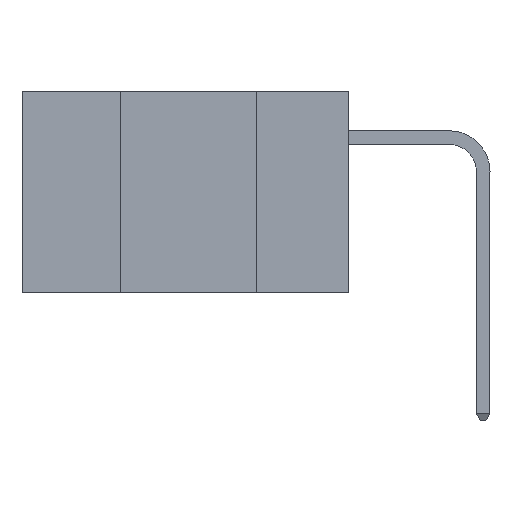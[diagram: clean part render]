
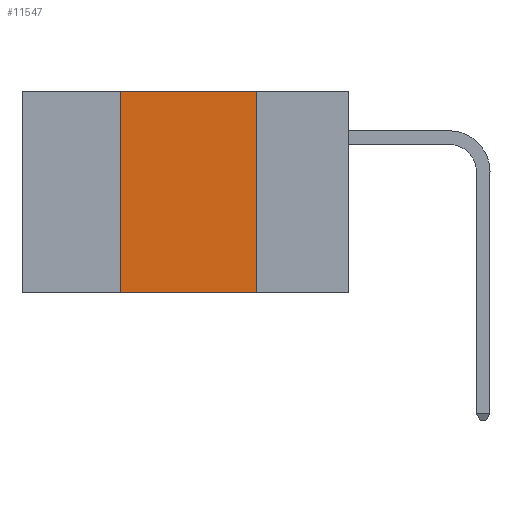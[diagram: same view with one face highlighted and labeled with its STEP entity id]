
A CAD part, left-side view. The second image highlights one B-rep face of the part: STEP entity #11547.
In plain terms, the highlighted planar face has unit normal (-1, 0, 0).
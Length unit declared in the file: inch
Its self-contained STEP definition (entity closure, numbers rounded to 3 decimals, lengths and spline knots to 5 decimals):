
#123 = CARTESIAN_POINT ( 'NONE',  ( 0., 0.42, -0.37 ) ) ;
#1362 = EDGE_LOOP ( 'NONE', ( #5322, #5265, #21734, #24463 ) ) ;
#3909 = EDGE_CURVE ( 'NONE', #28361, #12414, #17825, .T. ) ;
#4504 = CARTESIAN_POINT ( 'NONE',  ( 0., 0.17, 0. ) ) ;
#5265 = ORIENTED_EDGE ( 'NONE', *, *, #24788, .F. ) ;
#5299 = DIRECTION ( 'NONE',  ( 0., -1., 0. ) ) ;
#5322 = ORIENTED_EDGE ( 'NONE', *, *, #19753, .F. ) ;
#5754 = LINE ( 'NONE', #4504, #25176 ) ;
#6226 = DIRECTION ( 'NONE',  ( 0., 0., -1. ) ) ;
#8968 = VECTOR ( 'NONE', #5299, 39.37008 ) ;
#9313 = LINE ( 'NONE', #18518, #18513 ) ;
#11547 = ADVANCED_FACE ( 'NONE', ( #25370 ), #17026, .F. ) ;
#11687 = VERTEX_POINT ( 'NONE', #18327 ) ;
#12092 = DIRECTION ( 'NONE',  ( 0., -1., 0. ) ) ;
#12147 = CARTESIAN_POINT ( 'NONE',  ( 0., 0.42, 0. ) ) ;
#12414 = VERTEX_POINT ( 'NONE', #16113 ) ;
#12415 = CARTESIAN_POINT ( 'NONE',  ( 0., 0.17, 0. ) ) ;
#12488 = EDGE_CURVE ( 'NONE', #28361, #11687, #12990, .T. ) ;
#12990 = LINE ( 'NONE', #12147, #13978 ) ;
#13978 = VECTOR ( 'NONE', #16512, 39.37008 ) ;
#16113 = CARTESIAN_POINT ( 'NONE',  ( 0., 0.17, -0.37 ) ) ;
#16512 = DIRECTION ( 'NONE',  ( 0., 0., 1. ) ) ;
#17026 = PLANE ( 'NONE',  #27450 ) ;
#17231 = DIRECTION ( 'NONE',  ( 1., 0., 0. ) ) ;
#17825 = LINE ( 'NONE', #28169, #8968 ) ;
#18327 = CARTESIAN_POINT ( 'NONE',  ( 0., 0.42, 0. ) ) ;
#18513 = VECTOR ( 'NONE', #12092, 39.37008 ) ;
#18518 = CARTESIAN_POINT ( 'NONE',  ( 0., 0.6, 0. ) ) ;
#19753 = EDGE_CURVE ( 'NONE', #20171, #12414, #5754, .T. ) ;
#20171 = VERTEX_POINT ( 'NONE', #12415 ) ;
#20357 = DIRECTION ( 'NONE',  ( 0., 0., -1. ) ) ;
#21734 = ORIENTED_EDGE ( 'NONE', *, *, #12488, .F. ) ;
#24463 = ORIENTED_EDGE ( 'NONE', *, *, #3909, .T. ) ;
#24788 = EDGE_CURVE ( 'NONE', #11687, #20171, #9313, .T. ) ;
#25176 = VECTOR ( 'NONE', #20357, 39.37008 ) ;
#25370 = FACE_OUTER_BOUND ( 'NONE', #1362, .T. ) ;
#27450 = AXIS2_PLACEMENT_3D ( 'NONE', #28808, #17231, #6226 ) ;
#28169 = CARTESIAN_POINT ( 'NONE',  ( 0., 0.6, -0.37 ) ) ;
#28361 = VERTEX_POINT ( 'NONE', #123 ) ;
#28808 = CARTESIAN_POINT ( 'NONE',  ( 0., 0.6, 0. ) ) ;
